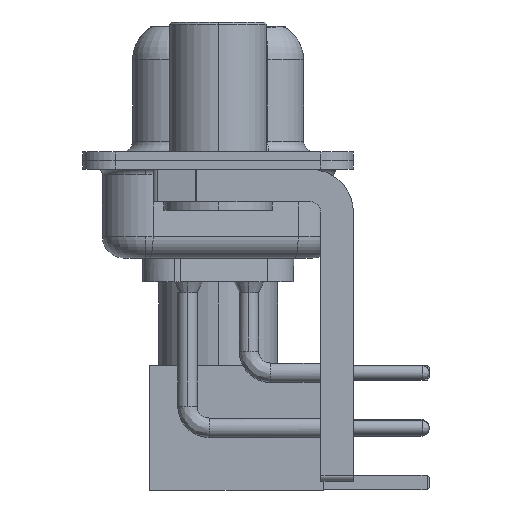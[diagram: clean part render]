
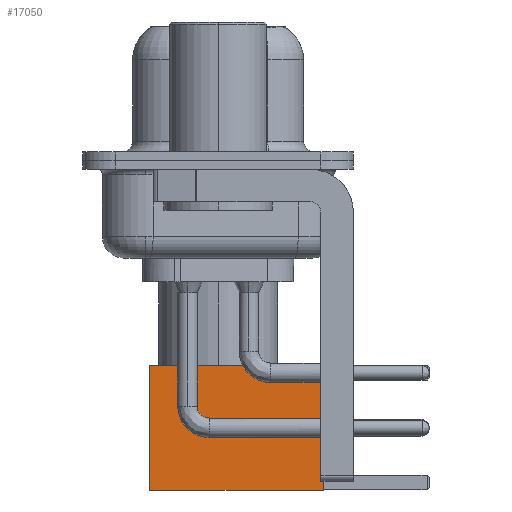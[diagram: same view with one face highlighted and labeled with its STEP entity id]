
A CAD part, left-side view. The second image highlights one B-rep face of the part: STEP entity #17050.
In plain terms, the highlighted face is planar.
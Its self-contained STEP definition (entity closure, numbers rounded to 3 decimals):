
#573 = LINE ( 'NONE', #26469, #22017 ) ;
#1206 = DIRECTION ( 'NONE',  ( 0., 0., 1. ) ) ;
#2015 = CARTESIAN_POINT ( 'NONE',  ( -2.875, 2.875, 0. ) ) ;
#3200 = LINE ( 'NONE', #2015, #23117 ) ;
#3838 = DIRECTION ( 'NONE',  ( -1., 0., 0. ) ) ;
#4061 = EDGE_CURVE ( 'NONE', #16123, #14994, #573, .T. ) ;
#4563 = ORIENTED_EDGE ( 'NONE', *, *, #7660, .T. ) ;
#5324 = CARTESIAN_POINT ( 'NONE',  ( -2.875, 2.875, 0. ) ) ;
#6144 = CARTESIAN_POINT ( 'NONE',  ( 0., 2.875, 0. ) ) ;
#6309 = DIRECTION ( 'NONE',  ( 0., 1., 0. ) ) ;
#7660 = EDGE_CURVE ( 'NONE', #24854, #21788, #27913, .T. ) ;
#7662 = LINE ( 'NONE', #20538, #23806 ) ;
#7912 = FACE_OUTER_BOUND ( 'NONE', #19977, .T. ) ;
#8559 = ORIENTED_EDGE ( 'NONE', *, *, #25688, .T. ) ;
#9915 = PLANE ( 'NONE',  #18533 ) ;
#14453 = CARTESIAN_POINT ( 'NONE',  ( 2.875, 2.875, 0. ) ) ;
#14994 = VERTEX_POINT ( 'NONE', #17202 ) ;
#16123 = VERTEX_POINT ( 'NONE', #19417 ) ;
#17050 = ADVANCED_FACE ( 'NONE', ( #7912 ), #9915, .T. ) ;
#17083 = EDGE_CURVE ( 'NONE', #14994, #21788, #3200, .T. ) ;
#17202 = CARTESIAN_POINT ( 'NONE',  ( -2.875, 2.875, 8. ) ) ;
#17281 = VECTOR ( 'NONE', #3838, 1000. ) ;
#17993 = ORIENTED_EDGE ( 'NONE', *, *, #4061, .F. ) ;
#18304 = DIRECTION ( 'NONE',  ( -1., 0., 0. ) ) ;
#18533 = AXIS2_PLACEMENT_3D ( 'NONE', #18653, #6309, #1206 ) ;
#18653 = CARTESIAN_POINT ( 'NONE',  ( 2.875, 2.875, 0. ) ) ;
#19417 = CARTESIAN_POINT ( 'NONE',  ( 2.875, 2.875, 8. ) ) ;
#19977 = EDGE_LOOP ( 'NONE', ( #8559, #4563, #23966, #17993 ) ) ;
#20538 = CARTESIAN_POINT ( 'NONE',  ( 2.875, 2.875, 0. ) ) ;
#21788 = VERTEX_POINT ( 'NONE', #5324 ) ;
#22017 = VECTOR ( 'NONE', #18304, 1000. ) ;
#23117 = VECTOR ( 'NONE', #23245, 1000. ) ;
#23245 = DIRECTION ( 'NONE',  ( 0., 0., -1. ) ) ;
#23806 = VECTOR ( 'NONE', #25138, 1000. ) ;
#23966 = ORIENTED_EDGE ( 'NONE', *, *, #17083, .F. ) ;
#24854 = VERTEX_POINT ( 'NONE', #14453 ) ;
#25138 = DIRECTION ( 'NONE',  ( 0., 0., -1. ) ) ;
#25688 = EDGE_CURVE ( 'NONE', #16123, #24854, #7662, .T. ) ;
#26469 = CARTESIAN_POINT ( 'NONE',  ( 0., 2.875, 8. ) ) ;
#27913 = LINE ( 'NONE', #6144, #17281 ) ;
